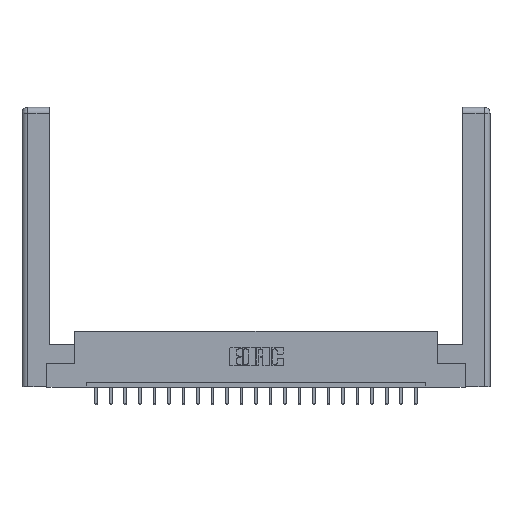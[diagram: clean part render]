
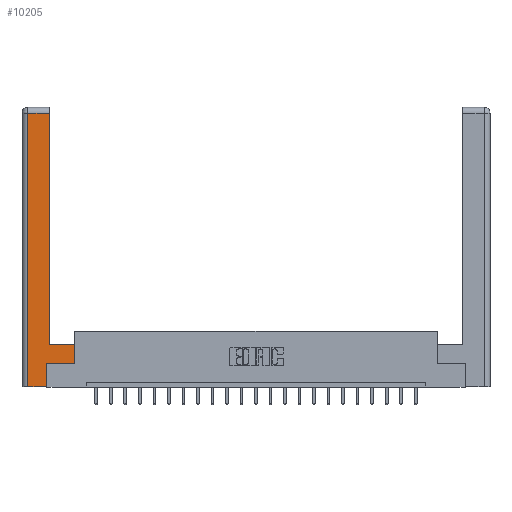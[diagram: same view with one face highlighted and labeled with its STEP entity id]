
A CAD part, top view. The second image highlights one B-rep face of the part: STEP entity #10205.
In plain terms, the highlighted planar face has unit normal (0, 0, 1).
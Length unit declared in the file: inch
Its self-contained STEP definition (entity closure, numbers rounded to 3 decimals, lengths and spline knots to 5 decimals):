
#132 = ORIENTED_EDGE ( 'NONE', *, *, #6717, .T. ) ;
#465 = DIRECTION ( 'NONE',  ( 0., 1., 0. ) ) ;
#1842 = DIRECTION ( 'NONE',  ( 0., -1., 0. ) ) ;
#2274 = ORIENTED_EDGE ( 'NONE', *, *, #18381, .T. ) ;
#2346 = EDGE_LOOP ( 'NONE', ( #2274, #16008, #132, #18704, #21736, #15999, #9391, #16918 ) ) ;
#2432 = CARTESIAN_POINT ( 'NONE',  ( 0.0615, 2.94, 0. ) ) ;
#2892 = VERTEX_POINT ( 'NONE', #10789 ) ;
#3258 = EDGE_CURVE ( 'NONE', #13304, #2892, #19383, .T. ) ;
#3622 = VECTOR ( 'NONE', #7375, 39.37008 ) ;
#4260 = PLANE ( 'NONE',  #21470 ) ;
#4937 = FACE_OUTER_BOUND ( 'NONE', #2346, .T. ) ;
#5222 = EDGE_CURVE ( 'NONE', #9390, #20033, #5809, .T. ) ;
#5574 = CARTESIAN_POINT ( 'NONE',  ( 0.565, 0.45, 0. ) ) ;
#5770 = CARTESIAN_POINT ( 'NONE',  ( 0.295, 0.45, 0. ) ) ;
#5809 = LINE ( 'NONE', #9211, #3622 ) ;
#5814 = VECTOR ( 'NONE', #13320, 39.37008 ) ;
#6563 = CARTESIAN_POINT ( 'NONE',  ( 0.0615, 0., 0. ) ) ;
#6717 = EDGE_CURVE ( 'NONE', #13005, #9390, #22289, .T. ) ;
#7114 = VERTEX_POINT ( 'NONE', #8988 ) ;
#7375 = DIRECTION ( 'NONE',  ( 1., 0., 0. ) ) ;
#7826 = EDGE_CURVE ( 'NONE', #17073, #13304, #15231, .T. ) ;
#7958 = VERTEX_POINT ( 'NONE', #16915 ) ;
#8333 = EDGE_CURVE ( 'NONE', #20033, #7114, #9039, .T. ) ;
#8482 = LINE ( 'NONE', #21049, #9026 ) ;
#8988 = CARTESIAN_POINT ( 'NONE',  ( 0.265, 0.245, 0. ) ) ;
#9026 = VECTOR ( 'NONE', #15771, 39.37008 ) ;
#9039 = LINE ( 'NONE', #21163, #21974 ) ;
#9211 = CARTESIAN_POINT ( 'NONE',  ( 0.265, 0., 0. ) ) ;
#9390 = VERTEX_POINT ( 'NONE', #6563 ) ;
#9391 = ORIENTED_EDGE ( 'NONE', *, *, #7826, .T. ) ;
#10205 = ADVANCED_FACE ( 'NONE', ( #4937 ), #4260, .F. ) ;
#10459 = CARTESIAN_POINT ( 'NONE',  ( 0.0615, 0., 0. ) ) ;
#10660 = VECTOR ( 'NONE', #18429, 39.37008 ) ;
#10789 = CARTESIAN_POINT ( 'NONE',  ( 0.295, 0.45, 0. ) ) ;
#11138 = DIRECTION ( 'NONE',  ( -1., 0., 0. ) ) ;
#11586 = CARTESIAN_POINT ( 'NONE',  ( 0.565, 0.45, 0. ) ) ;
#12349 = VECTOR ( 'NONE', #16614, 39.37008 ) ;
#12670 = DIRECTION ( 'NONE',  ( 0., 0., -1. ) ) ;
#13005 = VERTEX_POINT ( 'NONE', #2432 ) ;
#13154 = VECTOR ( 'NONE', #1842, 39.37008 ) ;
#13304 = VERTEX_POINT ( 'NONE', #5574 ) ;
#13320 = DIRECTION ( 'NONE',  ( 1., 0., 0. ) ) ;
#14372 = CARTESIAN_POINT ( 'NONE',  ( 0., 0., 0. ) ) ;
#14887 = CARTESIAN_POINT ( 'NONE',  ( 0.295, 3., 0. ) ) ;
#15231 = LINE ( 'NONE', #11586, #10660 ) ;
#15547 = LINE ( 'NONE', #21745, #5814 ) ;
#15771 = DIRECTION ( 'NONE',  ( -1., 0., 0. ) ) ;
#15999 = ORIENTED_EDGE ( 'NONE', *, *, #18352, .T. ) ;
#16008 = ORIENTED_EDGE ( 'NONE', *, *, #18641, .T. ) ;
#16247 = CARTESIAN_POINT ( 'NONE',  ( 0.565, 0.245, 0. ) ) ;
#16614 = DIRECTION ( 'NONE',  ( 0., 1., 0. ) ) ;
#16915 = CARTESIAN_POINT ( 'NONE',  ( 0.295, 2.94, 0. ) ) ;
#16918 = ORIENTED_EDGE ( 'NONE', *, *, #3258, .T. ) ;
#17073 = VERTEX_POINT ( 'NONE', #16247 ) ;
#18352 = EDGE_CURVE ( 'NONE', #7114, #17073, #15547, .T. ) ;
#18381 = EDGE_CURVE ( 'NONE', #2892, #7958, #19112, .T. ) ;
#18429 = DIRECTION ( 'NONE',  ( 0., 1., 0. ) ) ;
#18641 = EDGE_CURVE ( 'NONE', #7958, #13005, #8482, .T. ) ;
#18704 = ORIENTED_EDGE ( 'NONE', *, *, #5222, .T. ) ;
#19112 = LINE ( 'NONE', #14887, #12349 ) ;
#19383 = LINE ( 'NONE', #5770, #19915 ) ;
#19703 = DIRECTION ( 'NONE',  ( -1., 0., 0. ) ) ;
#19915 = VECTOR ( 'NONE', #11138, 39.37008 ) ;
#20033 = VERTEX_POINT ( 'NONE', #22306 ) ;
#21049 = CARTESIAN_POINT ( 'NONE',  ( 0.0615, 2.94, 0. ) ) ;
#21163 = CARTESIAN_POINT ( 'NONE',  ( 0.265, 0.245, 0. ) ) ;
#21470 = AXIS2_PLACEMENT_3D ( 'NONE', #14372, #12670, #19703 ) ;
#21736 = ORIENTED_EDGE ( 'NONE', *, *, #8333, .T. ) ;
#21745 = CARTESIAN_POINT ( 'NONE',  ( 0.565, 0.245, 0. ) ) ;
#21974 = VECTOR ( 'NONE', #465, 39.37008 ) ;
#22289 = LINE ( 'NONE', #10459, #13154 ) ;
#22306 = CARTESIAN_POINT ( 'NONE',  ( 0.265, 0., 0. ) ) ;
